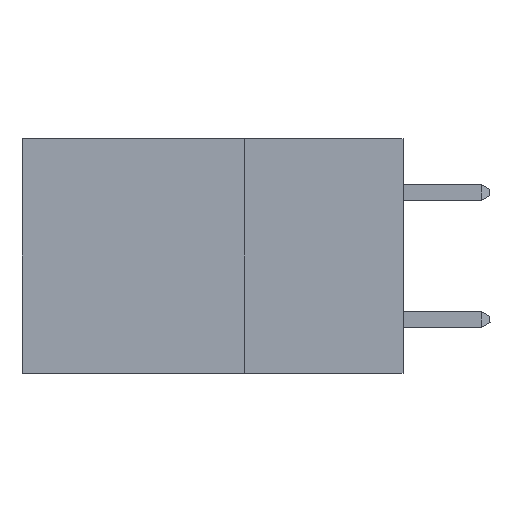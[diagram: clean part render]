
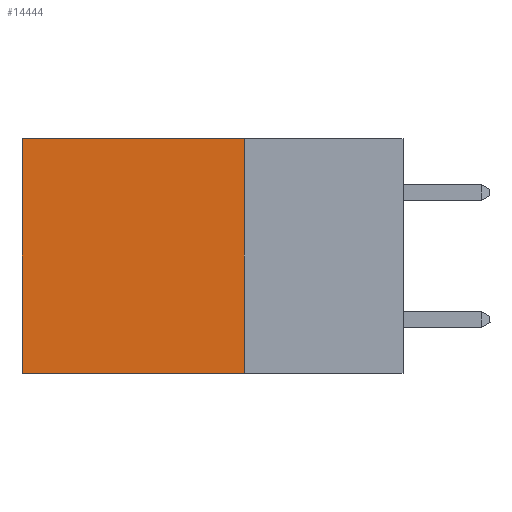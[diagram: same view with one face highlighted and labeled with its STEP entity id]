
A CAD part, left-side view. The second image highlights one B-rep face of the part: STEP entity #14444.
In plain terms, the highlighted planar face has unit normal (-1, 0, 0).
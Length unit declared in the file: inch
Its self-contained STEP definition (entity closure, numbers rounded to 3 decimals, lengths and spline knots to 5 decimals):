
#146 = VERTEX_POINT ( 'NONE', #35391 ) ;
#2387 = DIRECTION ( 'NONE',  ( 0., 1., 0. ) ) ;
#3559 = DIRECTION ( 'NONE',  ( 0., 0., -1. ) ) ;
#4637 = ORIENTED_EDGE ( 'NONE', *, *, #5592, .F. ) ;
#5592 = EDGE_CURVE ( 'NONE', #28347, #28405, #7836, .T. ) ;
#6790 = CARTESIAN_POINT ( 'NONE',  ( 0.2875, 0.25, -0.37 ) ) ;
#7836 = LINE ( 'NONE', #27609, #26065 ) ;
#8650 = ORIENTED_EDGE ( 'NONE', *, *, #37772, .T. ) ;
#10366 = CARTESIAN_POINT ( 'NONE',  ( 0.2875, 0.6, -0.37 ) ) ;
#13495 = LINE ( 'NONE', #17191, #39908 ) ;
#13615 = VERTEX_POINT ( 'NONE', #39003 ) ;
#14444 = ADVANCED_FACE ( 'NONE', ( #22689 ), #22477, .F. ) ;
#15584 = ORIENTED_EDGE ( 'NONE', *, *, #35002, .F. ) ;
#15902 = LINE ( 'NONE', #34479, #33145 ) ;
#17191 = CARTESIAN_POINT ( 'NONE',  ( 0.2875, 0.25, 0. ) ) ;
#19780 = DIRECTION ( 'NONE',  ( 1., 0., 0. ) ) ;
#20751 = DIRECTION ( 'NONE',  ( 0., 0., -1. ) ) ;
#22477 = PLANE ( 'NONE',  #30151 ) ;
#22689 = FACE_OUTER_BOUND ( 'NONE', #26483, .T. ) ;
#26065 = VECTOR ( 'NONE', #31064, 39.37008 ) ;
#26483 = EDGE_LOOP ( 'NONE', ( #8650, #4637, #15584, #42842 ) ) ;
#27609 = CARTESIAN_POINT ( 'NONE',  ( 0.2875, 0.25, -0.37 ) ) ;
#28347 = VERTEX_POINT ( 'NONE', #6790 ) ;
#28405 = VERTEX_POINT ( 'NONE', #10366 ) ;
#30151 = AXIS2_PLACEMENT_3D ( 'NONE', #33503, #19780, #43901 ) ;
#31064 = DIRECTION ( 'NONE',  ( 0., 1., 0. ) ) ;
#32384 = LINE ( 'NONE', #36820, #40497 ) ;
#33145 = VECTOR ( 'NONE', #20751, 39.37008 ) ;
#33503 = CARTESIAN_POINT ( 'NONE',  ( 0.2875, 0.25, 0. ) ) ;
#34479 = CARTESIAN_POINT ( 'NONE',  ( 0.2875, 0.6, 0. ) ) ;
#35002 = EDGE_CURVE ( 'NONE', #146, #28347, #13495, .T. ) ;
#35391 = CARTESIAN_POINT ( 'NONE',  ( 0.2875, 0.25, 0. ) ) ;
#36820 = CARTESIAN_POINT ( 'NONE',  ( 0.2875, 0.25, 0. ) ) ;
#37772 = EDGE_CURVE ( 'NONE', #13615, #28405, #15902, .T. ) ;
#39003 = CARTESIAN_POINT ( 'NONE',  ( 0.2875, 0.6, 0. ) ) ;
#39908 = VECTOR ( 'NONE', #3559, 39.37008 ) ;
#40497 = VECTOR ( 'NONE', #2387, 39.37008 ) ;
#40962 = EDGE_CURVE ( 'NONE', #146, #13615, #32384, .T. ) ;
#42842 = ORIENTED_EDGE ( 'NONE', *, *, #40962, .T. ) ;
#43901 = DIRECTION ( 'NONE',  ( 0., 0., -1. ) ) ;
